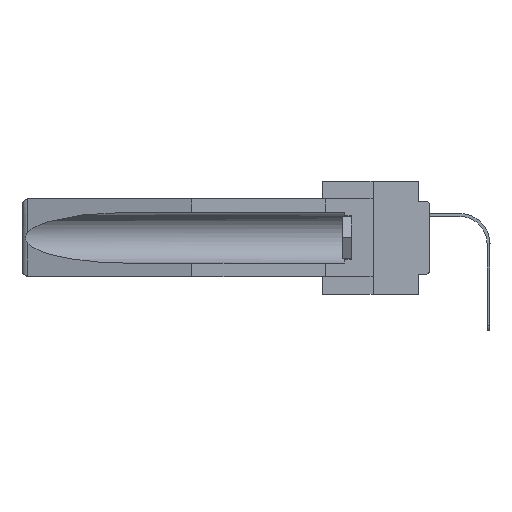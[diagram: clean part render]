
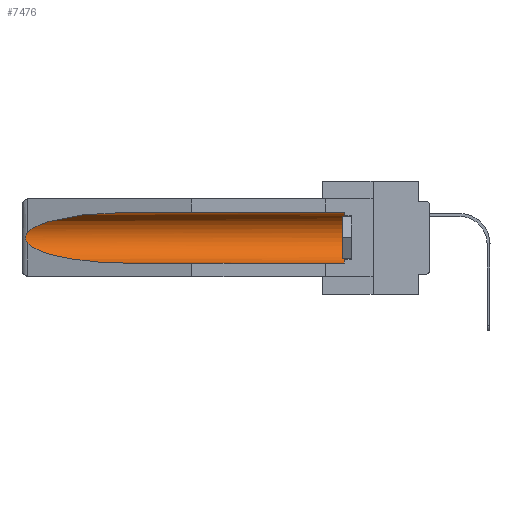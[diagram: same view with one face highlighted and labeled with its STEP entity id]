
A CAD part, left-side view. The second image highlights one B-rep face of the part: STEP entity #7476.
In plain terms, the highlighted cylindrical face has radius 2.857 mm (diameter 5.715 mm), a partial arc.
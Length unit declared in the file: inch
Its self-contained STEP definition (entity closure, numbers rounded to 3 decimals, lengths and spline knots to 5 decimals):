
#92 = DIRECTION ( 'NONE',  ( 0., 0., 1. ) ) ;
#342 = VECTOR ( 'NONE', #14083, 39.37008 ) ;
#381 = DIRECTION ( 'NONE',  ( 0., 0., 1. ) ) ;
#652 = VERTEX_POINT ( 'NONE', #28747 ) ;
#1123 = CARTESIAN_POINT ( 'NONE',  ( 0.2675, 1.53308, -0.17534 ) ) ;
#1302 = EDGE_CURVE ( 'NONE', #16631, #8508, #19591, .T. ) ;
#1391 = DIRECTION ( 'NONE',  ( 0., 1., 0. ) ) ;
#1546 = CARTESIAN_POINT ( 'NONE',  ( 0.155, 0.126, -0.284 ) ) ;
#4197 = CARTESIAN_POINT ( 'NONE',  ( 0.155, -0.30754, -0.284 ) ) ;
#4404 = CARTESIAN_POINT ( 'NONE',  ( 0.25451, 1.48313, -0.24835 ) ) ;
#4720 = CARTESIAN_POINT ( 'NONE',  ( 0.21114, 1.30732, -0.284 ) ) ;
#5560 = CARTESIAN_POINT ( 'NONE',  ( 0.155, -0.30754, -0.1715 ) ) ;
#6823 = CARTESIAN_POINT ( 'NONE',  ( 0.26537, 1.52718, -0.19328 ) ) ;
#7476 = ADVANCED_FACE ( 'NONE', ( #22211 ), #12540, .F. ) ;
#8072 = CARTESIAN_POINT ( 'NONE',  ( 0.2675, 1.53308, -0.16763 ) ) ;
#8219 = VERTEX_POINT ( 'NONE', #13063 ) ;
#8331 = EDGE_CURVE ( 'NONE', #8508, #22654, #21418, .T. ) ;
#8508 = VERTEX_POINT ( 'NONE', #29056 ) ;
#9090 = ORIENTED_EDGE ( 'NONE', *, *, #8331, .T. ) ;
#10997 = CARTESIAN_POINT ( 'NONE',  ( 0.26655, 1.53094, -0.18657 ) ) ;
#11884 = AXIS2_PLACEMENT_3D ( 'NONE', #24962, #22499, #381 ) ;
#12149 = CARTESIAN_POINT ( 'NONE',  ( 0.21114, 1.30732, -0.059 ) ) ;
#12540 = CYLINDRICAL_SURFACE ( 'NONE', #27354, 0.1125 ) ;
#13063 = CARTESIAN_POINT ( 'NONE',  ( 0.26537, 1.52718, -0.14972 ) ) ;
#13421 = CARTESIAN_POINT ( 'NONE',  ( 0.26597, 1.52961, -0.15275 ) ) ;
#14083 = DIRECTION ( 'NONE',  ( 0., 1., 0. ) ) ;
#14311 = CARTESIAN_POINT ( 'NONE',  ( 0.155, 1.07973, -0.059 ) ) ;
#16631 = VERTEX_POINT ( 'NONE', #1546 ) ;
#16836 = CARTESIAN_POINT ( 'NONE',  ( 0.155, 1.07973, -0.059 ) ) ;
#17157 = CARTESIAN_POINT ( 'NONE',  ( 0.155, 1.07973, -0.284 ) ) ;
#17172 = CARTESIAN_POINT ( 'NONE',  ( 0.155, 1.07973, -0.284 ) ) ;
#17597 = VECTOR ( 'NONE', #1391, 39.37008 ) ;
#17919 = CARTESIAN_POINT ( 'NONE',  ( 0.2673, 1.53269, -0.17917 ) ) ;
#18244 = CARTESIAN_POINT ( 'NONE',  ( 0.26537, 1.52718, -0.14972 ) ) ;
#18429 =( BOUNDED_CURVE ( )  B_SPLINE_CURVE ( 3, ( #16836, #12149, #28978, #21649 ),
 .UNSPECIFIED., .F., .F. ) 
 B_SPLINE_CURVE_WITH_KNOTS ( ( 4, 4 ),
 ( 4.71239, 6.08839 ),
 .UNSPECIFIED. ) 
 CURVE ( )  GEOMETRIC_REPRESENTATION_ITEM ( )  RATIONAL_B_SPLINE_CURVE ( ( 1., 0.848, 0.848, 1. ) ) 
 REPRESENTATION_ITEM ( '' )  );
#18771 = EDGE_CURVE ( 'NONE', #16631, #25566, #26343, .T. ) ;
#19591 = CIRCLE ( 'NONE', #11884, 0.1125 ) ;
#19660 = B_SPLINE_CURVE_WITH_KNOTS ( 'NONE', 3,
 ( #18244, #13421, #20350, #30239, #8072, #1123, #17919, #10997, #20818, #27789 ),
 .UNSPECIFIED., .F., .F.,
 ( 4, 2, 2, 2, 4 ),
 ( 0., 0.00029, 0.00058, 0.00087, 0.00117 ),
 .UNSPECIFIED. ) ;
#19873 = ORIENTED_EDGE ( 'NONE', *, *, #18771, .F. ) ;
#20350 = CARTESIAN_POINT ( 'NONE',  ( 0.26654, 1.53092, -0.15636 ) ) ;
#20818 = CARTESIAN_POINT ( 'NONE',  ( 0.26597, 1.5296, -0.19026 ) ) ;
#21117 = ORIENTED_EDGE ( 'NONE', *, *, #26927, .T. ) ;
#21418 = LINE ( 'NONE', #25801, #17597 ) ;
#21649 = CARTESIAN_POINT ( 'NONE',  ( 0.26537, 1.52718, -0.14972 ) ) ;
#21813 = EDGE_CURVE ( 'NONE', #22654, #8219, #18429, .T. ) ;
#22211 = FACE_OUTER_BOUND ( 'NONE', #29791, .T. ) ;
#22499 = DIRECTION ( 'NONE',  ( 0., -1., 0. ) ) ;
#22654 = VERTEX_POINT ( 'NONE', #14311 ) ;
#24463 = EDGE_CURVE ( 'NONE', #652, #25566, #25062, .T. ) ;
#24962 = CARTESIAN_POINT ( 'NONE',  ( 0.155, 0.126, -0.1715 ) ) ;
#25062 =( BOUNDED_CURVE ( )  B_SPLINE_CURVE ( 3, ( #6823, #4404, #4720, #17172 ),
 .UNSPECIFIED., .F., .F. ) 
 B_SPLINE_CURVE_WITH_KNOTS ( ( 4, 4 ),
 ( 0.1948, 1.5708 ),
 .UNSPECIFIED. ) 
 CURVE ( )  GEOMETRIC_REPRESENTATION_ITEM ( )  RATIONAL_B_SPLINE_CURVE ( ( 1., 0.848, 0.848, 1. ) ) 
 REPRESENTATION_ITEM ( '' )  );
#25566 = VERTEX_POINT ( 'NONE', #17157 ) ;
#25801 = CARTESIAN_POINT ( 'NONE',  ( 0.155, -0.30754, -0.059 ) ) ;
#26007 = ORIENTED_EDGE ( 'NONE', *, *, #24463, .T. ) ;
#26069 = ORIENTED_EDGE ( 'NONE', *, *, #21813, .T. ) ;
#26343 = LINE ( 'NONE', #4197, #342 ) ;
#26927 = EDGE_CURVE ( 'NONE', #8219, #652, #19660, .T. ) ;
#27354 = AXIS2_PLACEMENT_3D ( 'NONE', #5560, #30162, #92 ) ;
#27789 = CARTESIAN_POINT ( 'NONE',  ( 0.26537, 1.52718, -0.19328 ) ) ;
#28747 = CARTESIAN_POINT ( 'NONE',  ( 0.26537, 1.52718, -0.19328 ) ) ;
#28978 = CARTESIAN_POINT ( 'NONE',  ( 0.25451, 1.48313, -0.09465 ) ) ;
#29056 = CARTESIAN_POINT ( 'NONE',  ( 0.155, 0.126, -0.059 ) ) ;
#29791 = EDGE_LOOP ( 'NONE', ( #26069, #21117, #26007, #19873, #30247, #9090 ) ) ;
#30162 = DIRECTION ( 'NONE',  ( 0., 1., 0. ) ) ;
#30239 = CARTESIAN_POINT ( 'NONE',  ( 0.2673, 1.5327, -0.16383 ) ) ;
#30247 = ORIENTED_EDGE ( 'NONE', *, *, #1302, .T. ) ;
